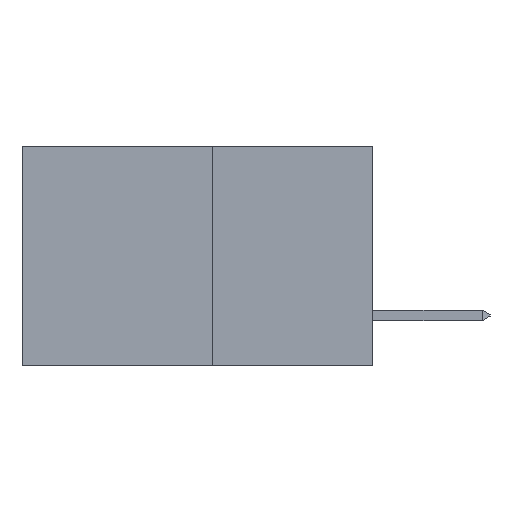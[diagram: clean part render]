
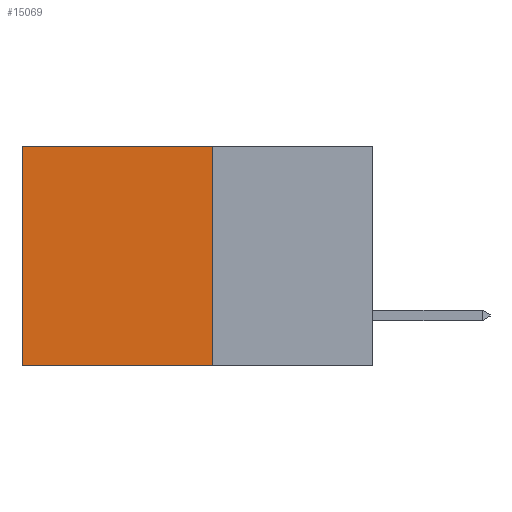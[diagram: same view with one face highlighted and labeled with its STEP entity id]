
A CAD part, left-side view. The second image highlights one B-rep face of the part: STEP entity #15069.
In plain terms, the highlighted planar face has unit normal (-1, 0, 0).
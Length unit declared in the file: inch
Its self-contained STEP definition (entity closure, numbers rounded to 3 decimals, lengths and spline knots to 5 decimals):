
#978 = LINE ( 'NONE', #3360, #4695 ) ;
#1555 = PLANE ( 'NONE',  #6592 ) ;
#2570 = DIRECTION ( 'NONE',  ( 0., 1., 0. ) ) ;
#3107 = CARTESIAN_POINT ( 'NONE',  ( 0.277, 0.27, -0.37 ) ) ;
#3360 = CARTESIAN_POINT ( 'NONE',  ( 0.277, 0.27, 0. ) ) ;
#3423 = DIRECTION ( 'NONE',  ( 1., 0., 0. ) ) ;
#3927 = CARTESIAN_POINT ( 'NONE',  ( 0.277, 0.27, 0. ) ) ;
#4513 = VERTEX_POINT ( 'NONE', #3927 ) ;
#4695 = VECTOR ( 'NONE', #2570, 39.37008 ) ;
#5268 = EDGE_CURVE ( 'NONE', #4513, #13764, #978, .T. ) ;
#6177 = CARTESIAN_POINT ( 'NONE',  ( 0.277, 0.27, -0.37 ) ) ;
#6554 = EDGE_LOOP ( 'NONE', ( #14865, #7318, #14750, #22733 ) ) ;
#6592 = AXIS2_PLACEMENT_3D ( 'NONE', #6978, #3423, #16043 ) ;
#6978 = CARTESIAN_POINT ( 'NONE',  ( 0.277, 0.27, -0.37 ) ) ;
#7318 = ORIENTED_EDGE ( 'NONE', *, *, #22838, .F. ) ;
#7372 = VERTEX_POINT ( 'NONE', #9348 ) ;
#7383 = VECTOR ( 'NONE', #20862, 39.37008 ) ;
#9348 = CARTESIAN_POINT ( 'NONE',  ( 0.277, 0.59, -0.37 ) ) ;
#9871 = DIRECTION ( 'NONE',  ( 0., 0., -1. ) ) ;
#11122 = LINE ( 'NONE', #6177, #20020 ) ;
#12216 = LINE ( 'NONE', #15531, #7383 ) ;
#12457 = CARTESIAN_POINT ( 'NONE',  ( 0.277, 0.59, -0.37 ) ) ;
#12746 = CARTESIAN_POINT ( 'NONE',  ( 0.277, 0.59, 0. ) ) ;
#13367 = EDGE_CURVE ( 'NONE', #4513, #18983, #11122, .T. ) ;
#13764 = VERTEX_POINT ( 'NONE', #12746 ) ;
#14257 = DIRECTION ( 'NONE',  ( 0., 0., -1. ) ) ;
#14346 = LINE ( 'NONE', #12457, #23128 ) ;
#14750 = ORIENTED_EDGE ( 'NONE', *, *, #13367, .F. ) ;
#14865 = ORIENTED_EDGE ( 'NONE', *, *, #17204, .T. ) ;
#15069 = ADVANCED_FACE ( 'NONE', ( #16647 ), #1555, .F. ) ;
#15531 = CARTESIAN_POINT ( 'NONE',  ( 0.277, 0.27, -0.37 ) ) ;
#16043 = DIRECTION ( 'NONE',  ( 0., 0., -1. ) ) ;
#16647 = FACE_OUTER_BOUND ( 'NONE', #6554, .T. ) ;
#17204 = EDGE_CURVE ( 'NONE', #13764, #7372, #14346, .T. ) ;
#18983 = VERTEX_POINT ( 'NONE', #3107 ) ;
#20020 = VECTOR ( 'NONE', #9871, 39.37008 ) ;
#20862 = DIRECTION ( 'NONE',  ( 0., 1., 0. ) ) ;
#22733 = ORIENTED_EDGE ( 'NONE', *, *, #5268, .T. ) ;
#22838 = EDGE_CURVE ( 'NONE', #18983, #7372, #12216, .T. ) ;
#23128 = VECTOR ( 'NONE', #14257, 39.37008 ) ;
